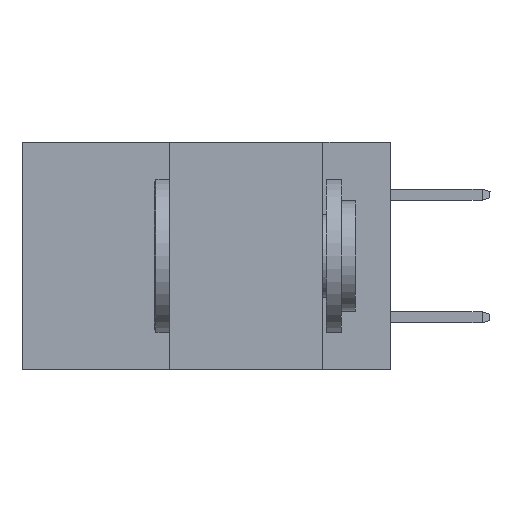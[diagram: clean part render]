
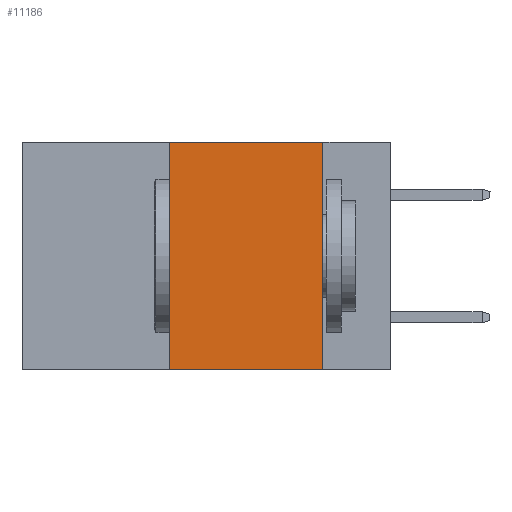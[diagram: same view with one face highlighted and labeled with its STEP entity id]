
A CAD part, left-side view. The second image highlights one B-rep face of the part: STEP entity #11186.
In plain terms, the highlighted planar face has unit normal (-1, 0, 0).
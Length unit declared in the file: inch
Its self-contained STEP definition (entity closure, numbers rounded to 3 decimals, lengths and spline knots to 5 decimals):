
#778 = LINE ( 'NONE', #5466, #2375 ) ;
#1619 = CARTESIAN_POINT ( 'NONE',  ( 0., 0.11, -0.37 ) ) ;
#1899 = DIRECTION ( 'NONE',  ( 0., 0., -1. ) ) ;
#2158 = EDGE_CURVE ( 'NONE', #3033, #18884, #4560, .T. ) ;
#2375 = VECTOR ( 'NONE', #12332, 39.37008 ) ;
#2571 = ORIENTED_EDGE ( 'NONE', *, *, #6786, .F. ) ;
#2881 = EDGE_CURVE ( 'NONE', #7374, #18049, #778, .T. ) ;
#3033 = VERTEX_POINT ( 'NONE', #20255 ) ;
#3153 = DIRECTION ( 'NONE',  ( 0., 0., -1. ) ) ;
#4560 = LINE ( 'NONE', #4830, #10194 ) ;
#4680 = ORIENTED_EDGE ( 'NONE', *, *, #2881, .T. ) ;
#4830 = CARTESIAN_POINT ( 'NONE',  ( 0., 0.6, 0. ) ) ;
#5466 = CARTESIAN_POINT ( 'NONE',  ( 0., 0.6, -0.37 ) ) ;
#5857 = CARTESIAN_POINT ( 'NONE',  ( 0., 0.11, 0. ) ) ;
#6589 = LINE ( 'NONE', #9910, #14108 ) ;
#6759 = EDGE_LOOP ( 'NONE', ( #16558, #11972, #2571, #4680 ) ) ;
#6786 = EDGE_CURVE ( 'NONE', #7374, #3033, #13747, .T. ) ;
#6853 = FACE_OUTER_BOUND ( 'NONE', #6759, .T. ) ;
#7374 = VERTEX_POINT ( 'NONE', #15786 ) ;
#8710 = DIRECTION ( 'NONE',  ( 1., 0., 0. ) ) ;
#8901 = VECTOR ( 'NONE', #12841, 39.37008 ) ;
#9215 = CARTESIAN_POINT ( 'NONE',  ( 0., 0.36, 0. ) ) ;
#9910 = CARTESIAN_POINT ( 'NONE',  ( 0., 0.11, 0. ) ) ;
#10077 = DIRECTION ( 'NONE',  ( 0., -1., 0. ) ) ;
#10194 = VECTOR ( 'NONE', #10077, 39.37008 ) ;
#11186 = ADVANCED_FACE ( 'NONE', ( #6853 ), #18821, .F. ) ;
#11650 = AXIS2_PLACEMENT_3D ( 'NONE', #18957, #8710, #1899 ) ;
#11972 = ORIENTED_EDGE ( 'NONE', *, *, #2158, .F. ) ;
#12332 = DIRECTION ( 'NONE',  ( 0., -1., 0. ) ) ;
#12841 = DIRECTION ( 'NONE',  ( 0., 0., 1. ) ) ;
#13747 = LINE ( 'NONE', #9215, #8901 ) ;
#14108 = VECTOR ( 'NONE', #3153, 39.37008 ) ;
#15786 = CARTESIAN_POINT ( 'NONE',  ( 0., 0.36, -0.37 ) ) ;
#16558 = ORIENTED_EDGE ( 'NONE', *, *, #20599, .F. ) ;
#18049 = VERTEX_POINT ( 'NONE', #1619 ) ;
#18821 = PLANE ( 'NONE',  #11650 ) ;
#18884 = VERTEX_POINT ( 'NONE', #5857 ) ;
#18957 = CARTESIAN_POINT ( 'NONE',  ( 0., 0.6, 0. ) ) ;
#20255 = CARTESIAN_POINT ( 'NONE',  ( 0., 0.36, 0. ) ) ;
#20599 = EDGE_CURVE ( 'NONE', #18884, #18049, #6589, .T. ) ;
